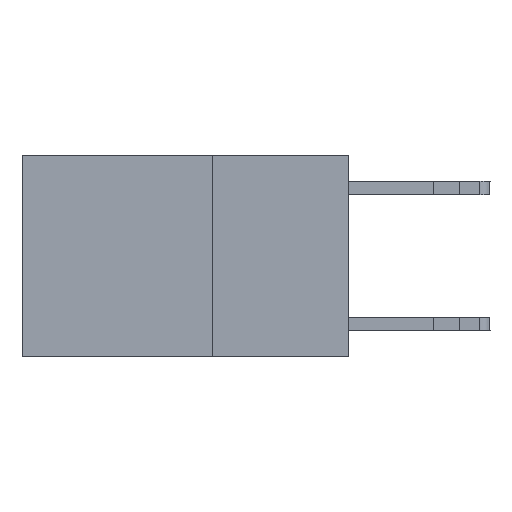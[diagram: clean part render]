
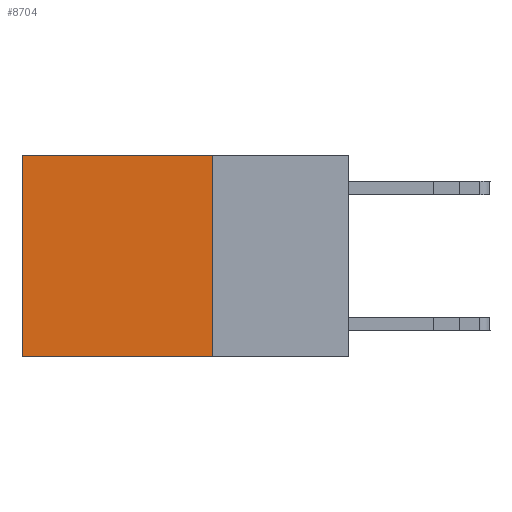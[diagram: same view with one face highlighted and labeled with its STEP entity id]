
A CAD part, left-side view. The second image highlights one B-rep face of the part: STEP entity #8704.
In plain terms, the highlighted planar face has unit normal (-1, 0, 0).
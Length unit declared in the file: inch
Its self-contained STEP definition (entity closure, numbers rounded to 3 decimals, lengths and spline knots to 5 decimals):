
#682 = CARTESIAN_POINT ( 'NONE',  ( 0.2625, 0.25, -0.37 ) ) ;
#1987 = EDGE_CURVE ( 'NONE', #3825, #10098, #6358, .T. ) ;
#3825 = VERTEX_POINT ( 'NONE', #21370 ) ;
#4638 = VECTOR ( 'NONE', #9477, 39.37008 ) ;
#4817 = CARTESIAN_POINT ( 'NONE',  ( 0.2625, 0.25, 0. ) ) ;
#6273 = VERTEX_POINT ( 'NONE', #16064 ) ;
#6358 = LINE ( 'NONE', #6470, #20921 ) ;
#6390 = LINE ( 'NONE', #8258, #16802 ) ;
#6470 = CARTESIAN_POINT ( 'NONE',  ( 0.2625, 0.25, 0. ) ) ;
#6672 = PLANE ( 'NONE',  #18946 ) ;
#7637 = LINE ( 'NONE', #21218, #4638 ) ;
#7821 = DIRECTION ( 'NONE',  ( 0., 1., 0. ) ) ;
#8131 = EDGE_LOOP ( 'NONE', ( #9678, #21038, #13285, #15805 ) ) ;
#8227 = DIRECTION ( 'NONE',  ( 0., 1., 0. ) ) ;
#8258 = CARTESIAN_POINT ( 'NONE',  ( 0.2625, 0.6, 0. ) ) ;
#8704 = ADVANCED_FACE ( 'NONE', ( #11604 ), #6672, .F. ) ;
#9477 = DIRECTION ( 'NONE',  ( 0., 0., -1. ) ) ;
#9678 = ORIENTED_EDGE ( 'NONE', *, *, #13689, .T. ) ;
#9792 = DIRECTION ( 'NONE',  ( 0., 0., -1. ) ) ;
#10098 = VERTEX_POINT ( 'NONE', #15140 ) ;
#11391 = DIRECTION ( 'NONE',  ( 0., 0., -1. ) ) ;
#11503 = DIRECTION ( 'NONE',  ( 1., 0., 0. ) ) ;
#11604 = FACE_OUTER_BOUND ( 'NONE', #8131, .T. ) ;
#13285 = ORIENTED_EDGE ( 'NONE', *, *, #15826, .F. ) ;
#13546 = EDGE_CURVE ( 'NONE', #16182, #6273, #15950, .T. ) ;
#13689 = EDGE_CURVE ( 'NONE', #10098, #6273, #6390, .T. ) ;
#15140 = CARTESIAN_POINT ( 'NONE',  ( 0.2625, 0.6, 0. ) ) ;
#15226 = VECTOR ( 'NONE', #7821, 39.37008 ) ;
#15805 = ORIENTED_EDGE ( 'NONE', *, *, #1987, .T. ) ;
#15826 = EDGE_CURVE ( 'NONE', #3825, #16182, #7637, .T. ) ;
#15950 = LINE ( 'NONE', #16062, #15226 ) ;
#16062 = CARTESIAN_POINT ( 'NONE',  ( 0.2625, 0.25, -0.37 ) ) ;
#16064 = CARTESIAN_POINT ( 'NONE',  ( 0.2625, 0.6, -0.37 ) ) ;
#16182 = VERTEX_POINT ( 'NONE', #682 ) ;
#16802 = VECTOR ( 'NONE', #9792, 39.37008 ) ;
#18946 = AXIS2_PLACEMENT_3D ( 'NONE', #4817, #11503, #11391 ) ;
#20921 = VECTOR ( 'NONE', #8227, 39.37008 ) ;
#21038 = ORIENTED_EDGE ( 'NONE', *, *, #13546, .F. ) ;
#21218 = CARTESIAN_POINT ( 'NONE',  ( 0.2625, 0.25, 0. ) ) ;
#21370 = CARTESIAN_POINT ( 'NONE',  ( 0.2625, 0.25, 0. ) ) ;
